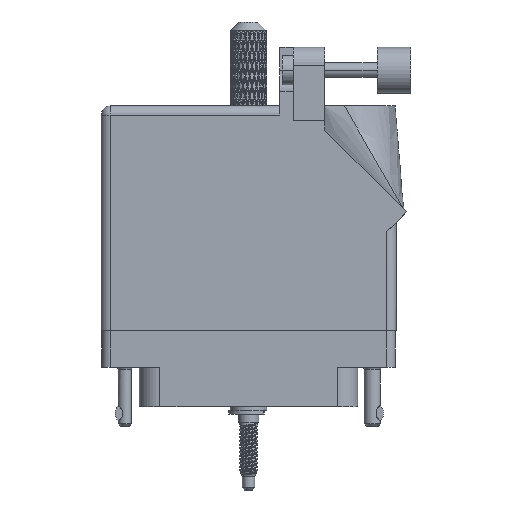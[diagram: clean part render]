
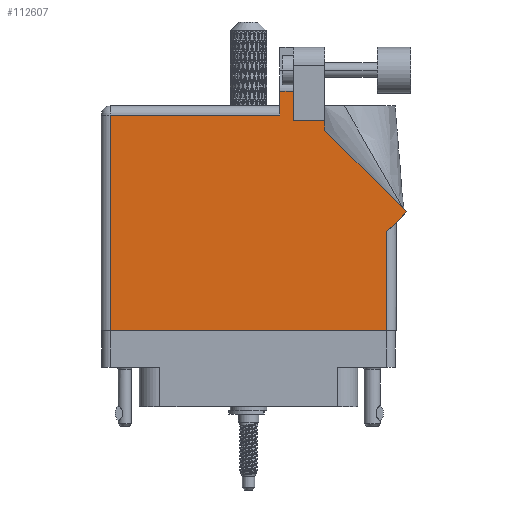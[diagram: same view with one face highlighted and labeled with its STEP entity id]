
A CAD part, front view. The second image highlights one B-rep face of the part: STEP entity #112607.
In plain terms, the highlighted face is planar.
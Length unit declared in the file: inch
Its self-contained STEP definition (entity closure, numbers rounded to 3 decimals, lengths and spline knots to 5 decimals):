
#900 = CARTESIAN_POINT ( 'NONE',  ( 1.07571, 0.70771, 0.455 ) ) ;
#5817 = VECTOR ( 'NONE', #37022, 39.37008 ) ;
#6033 = VERTEX_POINT ( 'NONE', #24936 ) ;
#9783 = DIRECTION ( 'NONE',  ( 0., 1., 0. ) ) ;
#11405 = DIRECTION ( 'NONE',  ( -0.707, 0.707, 0. ) ) ;
#12175 = EDGE_CURVE ( 'NONE', #25999, #34986, #20693, .T. ) ;
#12614 = CARTESIAN_POINT ( 'NONE',  ( 0.519, 1.26442, 0.455 ) ) ;
#13428 = VERTEX_POINT ( 'NONE', #48570 ) ;
#18489 = CARTESIAN_POINT ( 'NONE',  ( 0.519, 1.26442, 0.455 ) ) ;
#18765 = VERTEX_POINT ( 'NONE', #18767 ) ;
#18767 = CARTESIAN_POINT ( 'NONE',  ( 0.519, 1.33, 0.455 ) ) ;
#19515 = CARTESIAN_POINT ( 'NONE',  ( 0.306, 1.33, 0.455 ) ) ;
#20167 = LINE ( 'NONE', #55773, #94330 ) ;
#20302 = LINE ( 'NONE', #90357, #37776 ) ;
#20693 = LINE ( 'NONE', #53984, #87255 ) ;
#22070 = VERTEX_POINT ( 'NONE', #12614 ) ;
#23553 = VERTEX_POINT ( 'NONE', #98797 ) ;
#24059 = CARTESIAN_POINT ( 'NONE',  ( -0.943, 1.368, 0.455 ) ) ;
#24936 = CARTESIAN_POINT ( 'NONE',  ( -0.943, -0.1, 0.455 ) ) ;
#25999 = VERTEX_POINT ( 'NONE', #62981 ) ;
#26199 = EDGE_CURVE ( 'NONE', #96917, #6033, #56822, .T. ) ;
#28251 = VECTOR ( 'NONE', #9783, 39.37008 ) ;
#29000 = LINE ( 'NONE', #18489, #28251 ) ;
#29543 = ORIENTED_EDGE ( 'NONE', *, *, #55870, .T. ) ;
#32027 = EDGE_CURVE ( 'NONE', #98265, #13428, #72156, .T. ) ;
#32091 = ORIENTED_EDGE ( 'NONE', *, *, #62737, .T. ) ;
#32105 = ORIENTED_EDGE ( 'NONE', *, *, #93613, .T. ) ;
#33543 = EDGE_CURVE ( 'NONE', #18765, #112168, #95647, .T. ) ;
#34611 = VECTOR ( 'NONE', #43070, 39.37008 ) ;
#34632 = DIRECTION ( 'NONE',  ( 0., 0., -1. ) ) ;
#34950 = DIRECTION ( 'NONE',  ( 1., 0., 0. ) ) ;
#34986 = VERTEX_POINT ( 'NONE', #900 ) ;
#35163 = ORIENTED_EDGE ( 'NONE', *, *, #56670, .T. ) ;
#35384 = CARTESIAN_POINT ( 'NONE',  ( 0.63677, 1.5315, 0.455 ) ) ;
#35677 = VECTOR ( 'NONE', #34950, 39.37008 ) ;
#37022 = DIRECTION ( 'NONE',  ( 0., 1., 0. ) ) ;
#37776 = VECTOR ( 'NONE', #109072, 39.37008 ) ;
#39301 = CARTESIAN_POINT ( 'NONE',  ( 0.306, 1.5315, 0.455 ) ) ;
#39952 = ORIENTED_EDGE ( 'NONE', *, *, #32027, .T. ) ;
#40069 = VECTOR ( 'NONE', #71587, 39.37008 ) ;
#43070 = DIRECTION ( 'NONE',  ( -1., 0., 0. ) ) ;
#46220 = EDGE_CURVE ( 'NONE', #34986, #22070, #20167, .T. ) ;
#46773 = ORIENTED_EDGE ( 'NONE', *, *, #12175, .T. ) ;
#48105 = LINE ( 'NONE', #19515, #5817 ) ;
#48562 = ORIENTED_EDGE ( 'NONE', *, *, #33543, .T. ) ;
#48570 = CARTESIAN_POINT ( 'NONE',  ( 0.212, 1.5315, 0.455 ) ) ;
#50947 = ORIENTED_EDGE ( 'NONE', *, *, #26199, .T. ) ;
#51609 = CARTESIAN_POINT ( 'NONE',  ( -1.005, 1.43, 0.455 ) ) ;
#53984 = CARTESIAN_POINT ( 'NONE',  ( 1.005, 0.637, 0.455 ) ) ;
#55622 = VECTOR ( 'NONE', #60085, 39.37008 ) ;
#55773 = CARTESIAN_POINT ( 'NONE',  ( 1.07571, 0.70771, 0.455 ) ) ;
#55870 = EDGE_CURVE ( 'NONE', #13428, #23553, #115505, .T. ) ;
#56670 = EDGE_CURVE ( 'NONE', #66720, #25999, #110399, .T. ) ;
#56822 = LINE ( 'NONE', #90699, #65757 ) ;
#58363 = ORIENTED_EDGE ( 'NONE', *, *, #46220, .T. ) ;
#59382 = ORIENTED_EDGE ( 'NONE', *, *, #72111, .T. ) ;
#60085 = DIRECTION ( 'NONE',  ( 0., -1., 0. ) ) ;
#62737 = EDGE_CURVE ( 'NONE', #112168, #98265, #48105, .T. ) ;
#62981 = CARTESIAN_POINT ( 'NONE',  ( 0.943, 0.575, 0.455 ) ) ;
#65757 = VECTOR ( 'NONE', #72580, 39.37008 ) ;
#66720 = VERTEX_POINT ( 'NONE', #101026 ) ;
#71110 = CARTESIAN_POINT ( 'NONE',  ( 0.212, 1.43, 0.455 ) ) ;
#71587 = DIRECTION ( 'NONE',  ( -1., 0., 0. ) ) ;
#72111 = EDGE_CURVE ( 'NONE', #22070, #18765, #29000, .T. ) ;
#72156 = LINE ( 'NONE', #35384, #40069 ) ;
#72580 = DIRECTION ( 'NONE',  ( 0., -1., 0. ) ) ;
#73581 = DIRECTION ( 'NONE',  ( 0., 1., 0. ) ) ;
#73759 = ORIENTED_EDGE ( 'NONE', *, *, #99670, .T. ) ;
#76876 = EDGE_LOOP ( 'NONE', ( #32091, #39952, #29543, #73759, #50947, #32105, #35163, #46773, #58363, #59382, #48562 ) ) ;
#79009 = DIRECTION ( 'NONE',  ( -1., 0., 0. ) ) ;
#84053 = CARTESIAN_POINT ( 'NONE',  ( 0.943, 0.637, 0.455 ) ) ;
#87255 = VECTOR ( 'NONE', #89591, 39.37008 ) ;
#88579 = CARTESIAN_POINT ( 'NONE',  ( 0.519, 1.33, 0.455 ) ) ;
#89591 = DIRECTION ( 'NONE',  ( 0.707, 0.707, 0. ) ) ;
#90357 = CARTESIAN_POINT ( 'NONE',  ( -1.005, 1.368, 0.455 ) ) ;
#90699 = CARTESIAN_POINT ( 'NONE',  ( -0.943, -0.1, 0.455 ) ) ;
#93613 = EDGE_CURVE ( 'NONE', #6033, #66720, #114420, .T. ) ;
#94330 = VECTOR ( 'NONE', #11405, 39.37008 ) ;
#95647 = LINE ( 'NONE', #88579, #34611 ) ;
#96009 = PLANE ( 'NONE',  #105890 ) ;
#96917 = VERTEX_POINT ( 'NONE', #24059 ) ;
#98044 = CARTESIAN_POINT ( 'NONE',  ( 0.306, 1.33, 0.455 ) ) ;
#98265 = VERTEX_POINT ( 'NONE', #39301 ) ;
#98797 = CARTESIAN_POINT ( 'NONE',  ( 0.212, 1.368, 0.455 ) ) ;
#99670 = EDGE_CURVE ( 'NONE', #23553, #96917, #20302, .T. ) ;
#101026 = CARTESIAN_POINT ( 'NONE',  ( 0.943, -0.1, 0.455 ) ) ;
#105328 = FACE_OUTER_BOUND ( 'NONE', #76876, .T. ) ;
#105654 = CARTESIAN_POINT ( 'NONE',  ( -1.005, -0.1, 0.455 ) ) ;
#105890 = AXIS2_PLACEMENT_3D ( 'NONE', #51609, #34632, #79009 ) ;
#107897 = VECTOR ( 'NONE', #73581, 39.37008 ) ;
#109072 = DIRECTION ( 'NONE',  ( -1., 0., 0. ) ) ;
#110399 = LINE ( 'NONE', #84053, #107897 ) ;
#112168 = VERTEX_POINT ( 'NONE', #98044 ) ;
#112607 = ADVANCED_FACE ( 'NONE', ( #105328 ), #96009, .F. ) ;
#114420 = LINE ( 'NONE', #105654, #35677 ) ;
#115505 = LINE ( 'NONE', #71110, #55622 ) ;
